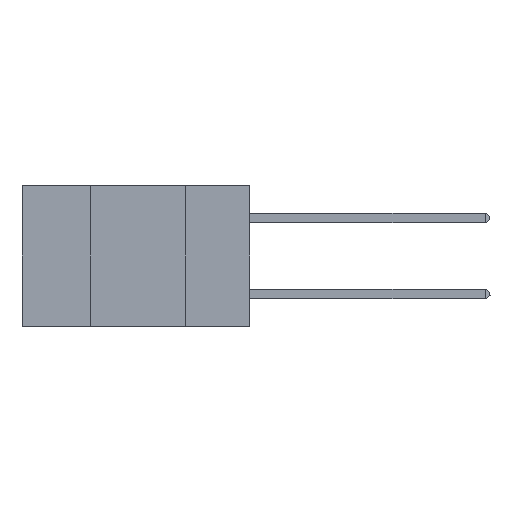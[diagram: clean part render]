
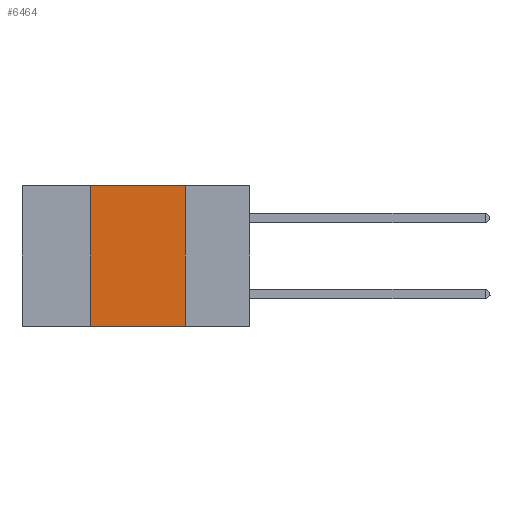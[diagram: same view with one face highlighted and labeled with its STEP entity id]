
A CAD part, left-side view. The second image highlights one B-rep face of the part: STEP entity #6464.
In plain terms, the highlighted planar face has unit normal (-1, 0, 0).
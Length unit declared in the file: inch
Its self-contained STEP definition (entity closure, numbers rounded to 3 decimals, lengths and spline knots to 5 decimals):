
#256 = EDGE_CURVE ( 'NONE', #10028, #20752, #9324, .T. ) ;
#576 = DIRECTION ( 'NONE',  ( 0., -1., 0. ) ) ;
#896 = ORIENTED_EDGE ( 'NONE', *, *, #256, .F. ) ;
#1655 = EDGE_CURVE ( 'NONE', #14285, #10028, #8231, .T. ) ;
#2087 = DIRECTION ( 'NONE',  ( 0., -1., 0. ) ) ;
#2237 = LINE ( 'NONE', #17444, #20457 ) ;
#2984 = ORIENTED_EDGE ( 'NONE', *, *, #7194, .F. ) ;
#3865 = EDGE_LOOP ( 'NONE', ( #2984, #896, #20243, #13977 ) ) ;
#4030 = CARTESIAN_POINT ( 'NONE',  ( 0., 0.17, 0. ) ) ;
#4279 = AXIS2_PLACEMENT_3D ( 'NONE', #11546, #14986, #16436 ) ;
#4818 = VECTOR ( 'NONE', #2087, 39.37008 ) ;
#5106 = CARTESIAN_POINT ( 'NONE',  ( 0., 0.42, -0.37 ) ) ;
#5738 = VECTOR ( 'NONE', #8820, 39.37008 ) ;
#6464 = ADVANCED_FACE ( 'NONE', ( #20578 ), #14769, .F. ) ;
#7145 = CARTESIAN_POINT ( 'NONE',  ( 0., 0.42, 0. ) ) ;
#7194 = EDGE_CURVE ( 'NONE', #20752, #13735, #13180, .T. ) ;
#7941 = DIRECTION ( 'NONE',  ( 0., 0., 1. ) ) ;
#8231 = LINE ( 'NONE', #21503, #11163 ) ;
#8741 = EDGE_CURVE ( 'NONE', #14285, #13735, #2237, .T. ) ;
#8820 = DIRECTION ( 'NONE',  ( 0., 0., -1. ) ) ;
#9324 = LINE ( 'NONE', #17382, #4818 ) ;
#10028 = VERTEX_POINT ( 'NONE', #7145 ) ;
#11163 = VECTOR ( 'NONE', #7941, 39.37008 ) ;
#11539 = CARTESIAN_POINT ( 'NONE',  ( 0., 0.17, 0. ) ) ;
#11546 = CARTESIAN_POINT ( 'NONE',  ( 0., 0.6, 0. ) ) ;
#13180 = LINE ( 'NONE', #4030, #5738 ) ;
#13735 = VERTEX_POINT ( 'NONE', #18944 ) ;
#13977 = ORIENTED_EDGE ( 'NONE', *, *, #8741, .T. ) ;
#14285 = VERTEX_POINT ( 'NONE', #5106 ) ;
#14769 = PLANE ( 'NONE',  #4279 ) ;
#14986 = DIRECTION ( 'NONE',  ( 1., 0., 0. ) ) ;
#16436 = DIRECTION ( 'NONE',  ( 0., 0., -1. ) ) ;
#17382 = CARTESIAN_POINT ( 'NONE',  ( 0., 0.6, 0. ) ) ;
#17444 = CARTESIAN_POINT ( 'NONE',  ( 0., 0.6, -0.37 ) ) ;
#18944 = CARTESIAN_POINT ( 'NONE',  ( 0., 0.17, -0.37 ) ) ;
#20243 = ORIENTED_EDGE ( 'NONE', *, *, #1655, .F. ) ;
#20457 = VECTOR ( 'NONE', #576, 39.37008 ) ;
#20578 = FACE_OUTER_BOUND ( 'NONE', #3865, .T. ) ;
#20752 = VERTEX_POINT ( 'NONE', #11539 ) ;
#21503 = CARTESIAN_POINT ( 'NONE',  ( 0., 0.42, 0. ) ) ;
